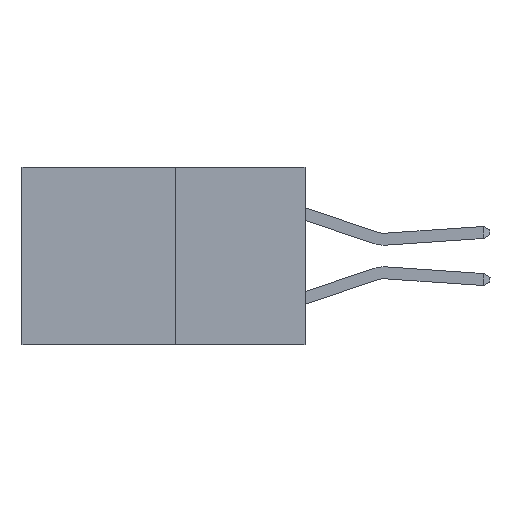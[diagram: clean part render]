
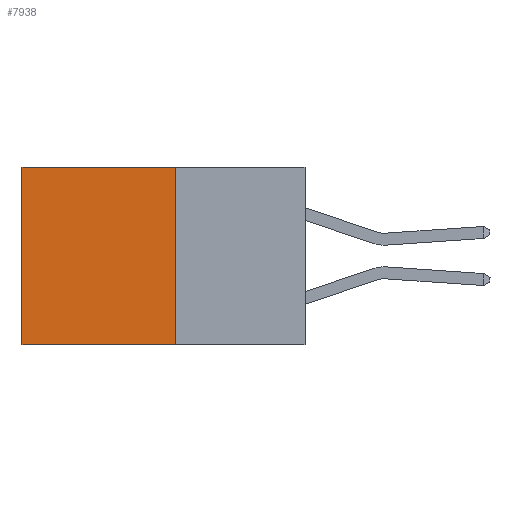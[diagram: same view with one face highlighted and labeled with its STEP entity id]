
A CAD part, left-side view. The second image highlights one B-rep face of the part: STEP entity #7938.
In plain terms, the highlighted planar face has unit normal (-1, 0, 0).
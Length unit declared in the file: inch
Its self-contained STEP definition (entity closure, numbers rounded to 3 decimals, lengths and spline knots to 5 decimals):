
#2628 = CARTESIAN_POINT ( 'NONE',  ( 0.277, 0.59, -0.37 ) ) ;
#3537 = VECTOR ( 'NONE', #22293, 39.37008 ) ;
#5367 = VERTEX_POINT ( 'NONE', #15939 ) ;
#6059 = LINE ( 'NONE', #19410, #11498 ) ;
#6195 = ORIENTED_EDGE ( 'NONE', *, *, #19032, .T. ) ;
#6230 = EDGE_LOOP ( 'NONE', ( #6195, #10827, #12079, #22872 ) ) ;
#6540 = DIRECTION ( 'NONE',  ( 0., 0., -1. ) ) ;
#6609 = DIRECTION ( 'NONE',  ( 1., 0., 0. ) ) ;
#6647 = PLANE ( 'NONE',  #20117 ) ;
#6652 = CARTESIAN_POINT ( 'NONE',  ( 0.277, 0.27, -0.37 ) ) ;
#7172 = EDGE_CURVE ( 'NONE', #13381, #26670, #10422, .T. ) ;
#7419 = DIRECTION ( 'NONE',  ( 0., 1., 0. ) ) ;
#7938 = ADVANCED_FACE ( 'NONE', ( #20790 ), #6647, .F. ) ;
#10422 = LINE ( 'NONE', #22495, #3537 ) ;
#10827 = ORIENTED_EDGE ( 'NONE', *, *, #7172, .F. ) ;
#11498 = VECTOR ( 'NONE', #21738, 39.37008 ) ;
#12079 = ORIENTED_EDGE ( 'NONE', *, *, #17351, .F. ) ;
#13381 = VERTEX_POINT ( 'NONE', #25724 ) ;
#13868 = CARTESIAN_POINT ( 'NONE',  ( 0.277, 0.59, -0.37 ) ) ;
#15634 = VECTOR ( 'NONE', #23351, 39.37008 ) ;
#15939 = CARTESIAN_POINT ( 'NONE',  ( 0.277, 0.59, 0. ) ) ;
#16284 = CARTESIAN_POINT ( 'NONE',  ( 0.277, 0.27, 0. ) ) ;
#16335 = LINE ( 'NONE', #2628, #15634 ) ;
#16380 = VERTEX_POINT ( 'NONE', #16284 ) ;
#17351 = EDGE_CURVE ( 'NONE', #16380, #13381, #6059, .T. ) ;
#18887 = CARTESIAN_POINT ( 'NONE',  ( 0.277, 0.27, 0. ) ) ;
#19032 = EDGE_CURVE ( 'NONE', #5367, #26670, #16335, .T. ) ;
#19410 = CARTESIAN_POINT ( 'NONE',  ( 0.277, 0.27, -0.37 ) ) ;
#20117 = AXIS2_PLACEMENT_3D ( 'NONE', #6652, #6609, #6540 ) ;
#20790 = FACE_OUTER_BOUND ( 'NONE', #6230, .T. ) ;
#20877 = LINE ( 'NONE', #18887, #26105 ) ;
#21738 = DIRECTION ( 'NONE',  ( 0., 0., -1. ) ) ;
#22293 = DIRECTION ( 'NONE',  ( 0., 1., 0. ) ) ;
#22495 = CARTESIAN_POINT ( 'NONE',  ( 0.277, 0.27, -0.37 ) ) ;
#22872 = ORIENTED_EDGE ( 'NONE', *, *, #26124, .T. ) ;
#23351 = DIRECTION ( 'NONE',  ( 0., 0., -1. ) ) ;
#25724 = CARTESIAN_POINT ( 'NONE',  ( 0.277, 0.27, -0.37 ) ) ;
#26105 = VECTOR ( 'NONE', #7419, 39.37008 ) ;
#26124 = EDGE_CURVE ( 'NONE', #16380, #5367, #20877, .T. ) ;
#26670 = VERTEX_POINT ( 'NONE', #13868 ) ;
